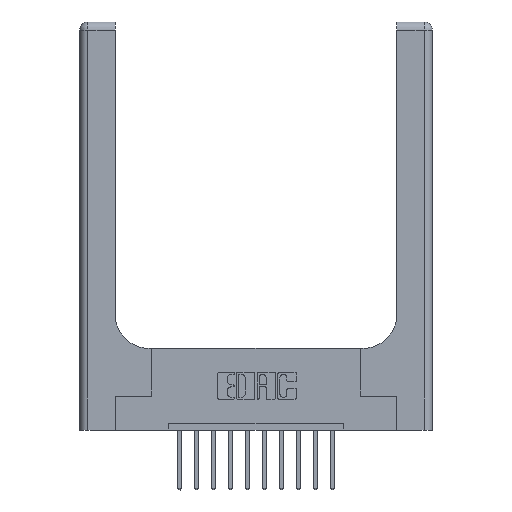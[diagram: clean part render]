
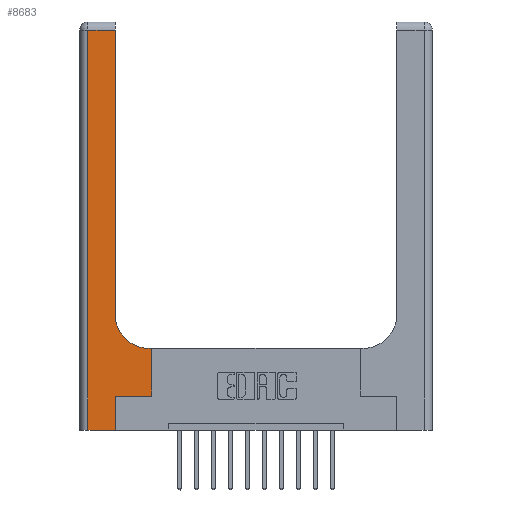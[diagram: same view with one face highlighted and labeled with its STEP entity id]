
A CAD part, top view. The second image highlights one B-rep face of the part: STEP entity #8683.
In plain terms, the highlighted planar face has unit normal (0, 0, 1).
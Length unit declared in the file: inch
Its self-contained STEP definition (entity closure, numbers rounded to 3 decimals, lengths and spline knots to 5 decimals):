
#608 = VECTOR ( 'NONE', #4291, 39.37008 ) ;
#649 = VECTOR ( 'NONE', #13669, 39.37008 ) ;
#886 = CARTESIAN_POINT ( 'NONE',  ( 0.06, 2.94, 0.37 ) ) ;
#1499 = LINE ( 'NONE', #7676, #4163 ) ;
#1753 = CARTESIAN_POINT ( 'NONE',  ( 0.51, 0.85, 0.37 ) ) ;
#2213 = DIRECTION ( 'NONE',  ( -1., 0., 0. ) ) ;
#2604 = LINE ( 'NONE', #6430, #6644 ) ;
#2733 = CARTESIAN_POINT ( 'NONE',  ( 0.265, 0.25, 0.37 ) ) ;
#2925 = EDGE_CURVE ( 'NONE', #12227, #10095, #1499, .T. ) ;
#3150 = ORIENTED_EDGE ( 'NONE', *, *, #12408, .T. ) ;
#3511 = VERTEX_POINT ( 'NONE', #13979 ) ;
#3526 = VERTEX_POINT ( 'NONE', #5462 ) ;
#3703 = ORIENTED_EDGE ( 'NONE', *, *, #12702, .T. ) ;
#4163 = VECTOR ( 'NONE', #5151, 39.37008 ) ;
#4238 = CARTESIAN_POINT ( 'NONE',  ( 0., 0., 0.37 ) ) ;
#4262 = VERTEX_POINT ( 'NONE', #13181 ) ;
#4284 = LINE ( 'NONE', #10740, #7196 ) ;
#4291 = DIRECTION ( 'NONE',  ( 1., 0., 0. ) ) ;
#4338 = EDGE_CURVE ( 'NONE', #4262, #14102, #6055, .T. ) ;
#4822 = VERTEX_POINT ( 'NONE', #13757 ) ;
#4887 = DIRECTION ( 'NONE',  ( -1., 0., 0. ) ) ;
#4891 = CIRCLE ( 'NONE', #11480, 0.25 ) ;
#5151 = DIRECTION ( 'NONE',  ( 0., 1., 0. ) ) ;
#5174 = VECTOR ( 'NONE', #6575, 39.37008 ) ;
#5462 = CARTESIAN_POINT ( 'NONE',  ( 0.26, 0.85, 0.37 ) ) ;
#5871 = AXIS2_PLACEMENT_3D ( 'NONE', #14386, #14239, #8239 ) ;
#5906 = PLANE ( 'NONE',  #5871 ) ;
#6010 = ORIENTED_EDGE ( 'NONE', *, *, #13012, .T. ) ;
#6055 = LINE ( 'NONE', #10969, #7967 ) ;
#6237 = ORIENTED_EDGE ( 'NONE', *, *, #11676, .T. ) ;
#6430 = CARTESIAN_POINT ( 'NONE',  ( 0.528, 0.25, 0.37 ) ) ;
#6575 = DIRECTION ( 'NONE',  ( 0., -1., 0. ) ) ;
#6644 = VECTOR ( 'NONE', #7649, 39.37008 ) ;
#6714 = CARTESIAN_POINT ( 'NONE',  ( 0.06, 0., 0.37 ) ) ;
#6865 = ORIENTED_EDGE ( 'NONE', *, *, #11576, .T. ) ;
#7139 = LINE ( 'NONE', #4238, #608 ) ;
#7196 = VECTOR ( 'NONE', #2213, 39.37008 ) ;
#7649 = DIRECTION ( 'NONE',  ( 0., 1., 0. ) ) ;
#7676 = CARTESIAN_POINT ( 'NONE',  ( 0.265, 0., 0.37 ) ) ;
#7952 = EDGE_CURVE ( 'NONE', #13375, #15513, #8435, .T. ) ;
#7967 = VECTOR ( 'NONE', #4887, 39.37008 ) ;
#8111 = LINE ( 'NONE', #2733, #649 ) ;
#8239 = DIRECTION ( 'NONE',  ( -1., 0., 0. ) ) ;
#8435 = LINE ( 'NONE', #8911, #5174 ) ;
#8683 = ADVANCED_FACE ( 'NONE', ( #8998 ), #5906, .F. ) ;
#8911 = CARTESIAN_POINT ( 'NONE',  ( 0.06, 3., 0.37 ) ) ;
#8998 = FACE_OUTER_BOUND ( 'NONE', #10549, .T. ) ;
#9755 = DIRECTION ( 'NONE',  ( 0., 1., 0. ) ) ;
#9968 = CARTESIAN_POINT ( 'NONE',  ( 0.26, 3., 0.37 ) ) ;
#10095 = VERTEX_POINT ( 'NONE', #10987 ) ;
#10299 = DIRECTION ( 'NONE',  ( 1., 0., 0. ) ) ;
#10395 = DIRECTION ( 'NONE',  ( 0., 0., -1. ) ) ;
#10549 = EDGE_LOOP ( 'NONE', ( #6010, #3150, #15195, #13285, #12015, #3703, #6865, #12166, #6237 ) ) ;
#10740 = CARTESIAN_POINT ( 'NONE',  ( 0., 2.94, 0.37 ) ) ;
#10969 = CARTESIAN_POINT ( 'NONE',  ( 0.26, 0.6, 0.37 ) ) ;
#10987 = CARTESIAN_POINT ( 'NONE',  ( 0.265, 0.25, 0.37 ) ) ;
#11480 = AXIS2_PLACEMENT_3D ( 'NONE', #1753, #10395, #10299 ) ;
#11499 = VECTOR ( 'NONE', #9755, 39.37008 ) ;
#11576 = EDGE_CURVE ( 'NONE', #3511, #4262, #2604, .T. ) ;
#11676 = EDGE_CURVE ( 'NONE', #14102, #3526, #4891, .T. ) ;
#11876 = LINE ( 'NONE', #9968, #11499 ) ;
#12015 = ORIENTED_EDGE ( 'NONE', *, *, #2925, .T. ) ;
#12166 = ORIENTED_EDGE ( 'NONE', *, *, #4338, .T. ) ;
#12227 = VERTEX_POINT ( 'NONE', #13636 ) ;
#12408 = EDGE_CURVE ( 'NONE', #4822, #13375, #4284, .T. ) ;
#12702 = EDGE_CURVE ( 'NONE', #10095, #3511, #8111, .T. ) ;
#13012 = EDGE_CURVE ( 'NONE', #3526, #4822, #11876, .T. ) ;
#13181 = CARTESIAN_POINT ( 'NONE',  ( 0.528, 0.6, 0.37 ) ) ;
#13285 = ORIENTED_EDGE ( 'NONE', *, *, #14887, .T. ) ;
#13375 = VERTEX_POINT ( 'NONE', #886 ) ;
#13636 = CARTESIAN_POINT ( 'NONE',  ( 0.265, 0., 0.37 ) ) ;
#13669 = DIRECTION ( 'NONE',  ( 1., 0., 0. ) ) ;
#13757 = CARTESIAN_POINT ( 'NONE',  ( 0.26, 2.94, 0.37 ) ) ;
#13979 = CARTESIAN_POINT ( 'NONE',  ( 0.528, 0.25, 0.37 ) ) ;
#14102 = VERTEX_POINT ( 'NONE', #15713 ) ;
#14239 = DIRECTION ( 'NONE',  ( 0., 0., -1. ) ) ;
#14386 = CARTESIAN_POINT ( 'NONE',  ( 0., 3., 0.37 ) ) ;
#14887 = EDGE_CURVE ( 'NONE', #15513, #12227, #7139, .T. ) ;
#15195 = ORIENTED_EDGE ( 'NONE', *, *, #7952, .T. ) ;
#15513 = VERTEX_POINT ( 'NONE', #6714 ) ;
#15713 = CARTESIAN_POINT ( 'NONE',  ( 0.51, 0.6, 0.37 ) ) ;
